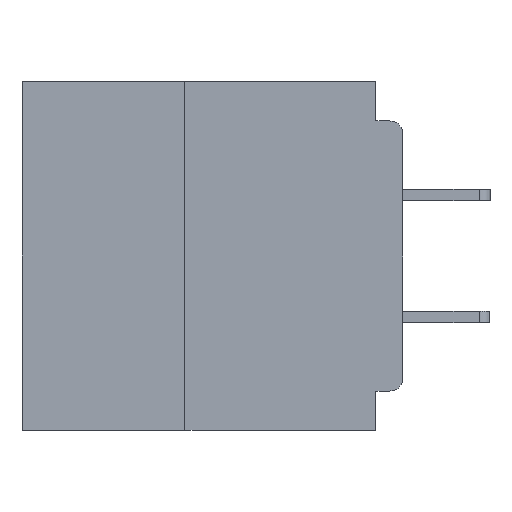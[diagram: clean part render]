
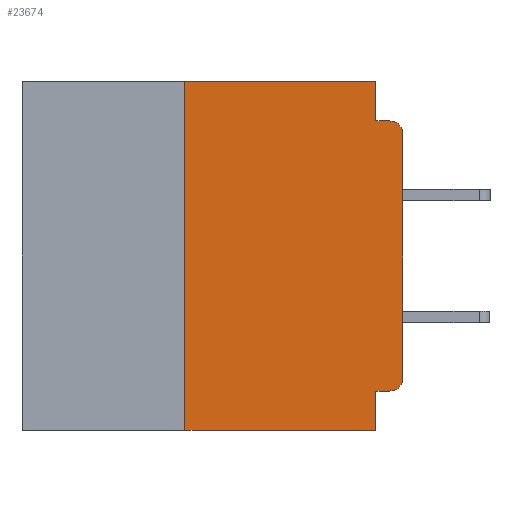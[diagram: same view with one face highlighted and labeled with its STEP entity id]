
A CAD part, left-side view. The second image highlights one B-rep face of the part: STEP entity #23674.
In plain terms, the highlighted planar face has unit normal (-1, 0, 0).
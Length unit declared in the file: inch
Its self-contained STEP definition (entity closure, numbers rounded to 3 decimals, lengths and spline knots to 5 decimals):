
#509 = VERTEX_POINT ( 'NONE', #4498 ) ;
#1173 = EDGE_CURVE ( 'NONE', #20851, #509, #19876, .T. ) ;
#1231 = DIRECTION ( 'NONE',  ( 0., -1., 0. ) ) ;
#1664 = DIRECTION ( 'NONE',  ( 0., 1., 0. ) ) ;
#2413 = DIRECTION ( 'NONE',  ( 0., 0., 1. ) ) ;
#2681 = CARTESIAN_POINT ( 'NONE',  ( 0., 0.015, -0.34 ) ) ;
#2806 = LINE ( 'NONE', #38036, #23431 ) ;
#3100 = CARTESIAN_POINT ( 'NONE',  ( 0., 0.031, 0. ) ) ;
#3431 = VERTEX_POINT ( 'NONE', #19432 ) ;
#4291 = CARTESIAN_POINT ( 'NONE',  ( 0., 0.031, -0.4 ) ) ;
#4498 = CARTESIAN_POINT ( 'NONE',  ( 0., 0.015, -0.045 ) ) ;
#4649 = VECTOR ( 'NONE', #23193, 39.37008 ) ;
#5058 = EDGE_CURVE ( 'NONE', #21320, #20851, #5651, .T. ) ;
#5164 = CARTESIAN_POINT ( 'NONE',  ( 0., 0., -0.045 ) ) ;
#5386 = DIRECTION ( 'NONE',  ( -1., 0., 0. ) ) ;
#5651 = LINE ( 'NONE', #7080, #36020 ) ;
#5816 = DIRECTION ( 'NONE',  ( 0., 0., -1. ) ) ;
#6652 = CARTESIAN_POINT ( 'NONE',  ( 0., 0.437, -0.4 ) ) ;
#6948 = DIRECTION ( 'NONE',  ( 0., 0., -1. ) ) ;
#7080 = CARTESIAN_POINT ( 'NONE',  ( 0., 0.031, 0. ) ) ;
#7902 = DIRECTION ( 'NONE',  ( 0., -1., 0. ) ) ;
#7942 = CARTESIAN_POINT ( 'NONE',  ( 0., 0., -0.06 ) ) ;
#8450 = CARTESIAN_POINT ( 'NONE',  ( 0., 0.25, -0.4 ) ) ;
#8512 = CARTESIAN_POINT ( 'NONE',  ( 0., 0., 0. ) ) ;
#8685 = VECTOR ( 'NONE', #1664, 39.37008 ) ;
#9757 = DIRECTION ( 'NONE',  ( 0., -1., 0. ) ) ;
#11208 = CARTESIAN_POINT ( 'NONE',  ( 0., 0., -0.34 ) ) ;
#12075 = EDGE_CURVE ( 'NONE', #3431, #20277, #26276, .T. ) ;
#12393 = VERTEX_POINT ( 'NONE', #4291 ) ;
#13292 = LINE ( 'NONE', #33837, #28543 ) ;
#13710 = CARTESIAN_POINT ( 'NONE',  ( 0., 0.25, 0. ) ) ;
#16105 = VERTEX_POINT ( 'NONE', #13710 ) ;
#16171 = VERTEX_POINT ( 'NONE', #7942 ) ;
#16771 = VECTOR ( 'NONE', #2413, 39.37008 ) ;
#16838 = LINE ( 'NONE', #35045, #8685 ) ;
#17306 = DIRECTION ( 'NONE',  ( 1., 0., 0. ) ) ;
#17730 = EDGE_CURVE ( 'NONE', #3431, #23678, #16838, .T. ) ;
#18476 = EDGE_CURVE ( 'NONE', #20277, #16171, #24841, .T. ) ;
#19432 = CARTESIAN_POINT ( 'NONE',  ( 0., 0.015, -0.355 ) ) ;
#19876 = LINE ( 'NONE', #5164, #20830 ) ;
#20163 = CARTESIAN_POINT ( 'NONE',  ( 0., 0.031, -0.4 ) ) ;
#20218 = EDGE_CURVE ( 'NONE', #23678, #12393, #28097, .T. ) ;
#20277 = VERTEX_POINT ( 'NONE', #11208 ) ;
#20287 = EDGE_LOOP ( 'NONE', ( #28439, #28703, #28789, #29119, #29197, #29611, #29644, #33508, #33580, #22448 ) ) ;
#20830 = VECTOR ( 'NONE', #1231, 39.37008 ) ;
#20851 = VERTEX_POINT ( 'NONE', #30638 ) ;
#21320 = VERTEX_POINT ( 'NONE', #3100 ) ;
#21760 = EDGE_CURVE ( 'NONE', #16171, #509, #24611, .T. ) ;
#22448 = ORIENTED_EDGE ( 'NONE', *, *, #12075, .T. ) ;
#23193 = DIRECTION ( 'NONE',  ( 0., 0., -1. ) ) ;
#23431 = VECTOR ( 'NONE', #7902, 39.37008 ) ;
#23674 = ADVANCED_FACE ( 'NONE', ( #37560 ), #32331, .F. ) ;
#23678 = VERTEX_POINT ( 'NONE', #35333 ) ;
#23711 = CARTESIAN_POINT ( 'NONE',  ( 0., 0.015, -0.06 ) ) ;
#23736 = VERTEX_POINT ( 'NONE', #8450 ) ;
#24116 = DIRECTION ( 'NONE',  ( -1., 0., 0. ) ) ;
#24458 = LINE ( 'NONE', #6652, #39407 ) ;
#24611 = CIRCLE ( 'NONE', #28596, 0.015 ) ;
#24841 = LINE ( 'NONE', #8512, #16771 ) ;
#26276 = CIRCLE ( 'NONE', #27075, 0.015 ) ;
#26329 = EDGE_CURVE ( 'NONE', #23736, #12393, #24458, .T. ) ;
#26776 = DIRECTION ( 'NONE',  ( 0., 0., -1. ) ) ;
#27075 = AXIS2_PLACEMENT_3D ( 'NONE', #2681, #24116, #5816 ) ;
#28097 = LINE ( 'NONE', #20163, #4649 ) ;
#28439 = ORIENTED_EDGE ( 'NONE', *, *, #18476, .T. ) ;
#28543 = VECTOR ( 'NONE', #36805, 39.37008 ) ;
#28596 = AXIS2_PLACEMENT_3D ( 'NONE', #23711, #5386, #26776 ) ;
#28703 = ORIENTED_EDGE ( 'NONE', *, *, #21760, .T. ) ;
#28789 = ORIENTED_EDGE ( 'NONE', *, *, #1173, .F. ) ;
#29119 = ORIENTED_EDGE ( 'NONE', *, *, #5058, .F. ) ;
#29197 = ORIENTED_EDGE ( 'NONE', *, *, #34301, .F. ) ;
#29387 = CARTESIAN_POINT ( 'NONE',  ( 0., 0.437, 0. ) ) ;
#29611 = ORIENTED_EDGE ( 'NONE', *, *, #30352, .F. ) ;
#29644 = ORIENTED_EDGE ( 'NONE', *, *, #26329, .T. ) ;
#30352 = EDGE_CURVE ( 'NONE', #23736, #16105, #13292, .T. ) ;
#30638 = CARTESIAN_POINT ( 'NONE',  ( 0., 0.031, -0.045 ) ) ;
#32331 = PLANE ( 'NONE',  #35553 ) ;
#33508 = ORIENTED_EDGE ( 'NONE', *, *, #20218, .F. ) ;
#33580 = ORIENTED_EDGE ( 'NONE', *, *, #17730, .F. ) ;
#33837 = CARTESIAN_POINT ( 'NONE',  ( 0., 0.25, -0.4 ) ) ;
#34301 = EDGE_CURVE ( 'NONE', #16105, #21320, #2806, .T. ) ;
#35045 = CARTESIAN_POINT ( 'NONE',  ( 0., 0., -0.355 ) ) ;
#35333 = CARTESIAN_POINT ( 'NONE',  ( 0., 0.031, -0.355 ) ) ;
#35553 = AXIS2_PLACEMENT_3D ( 'NONE', #29387, #17306, #38288 ) ;
#36020 = VECTOR ( 'NONE', #6948, 39.37008 ) ;
#36805 = DIRECTION ( 'NONE',  ( 0., 0., 1. ) ) ;
#37560 = FACE_OUTER_BOUND ( 'NONE', #20287, .T. ) ;
#38036 = CARTESIAN_POINT ( 'NONE',  ( 0., 0.437, 0. ) ) ;
#38288 = DIRECTION ( 'NONE',  ( 0., 0., -1. ) ) ;
#39407 = VECTOR ( 'NONE', #9757, 39.37008 ) ;
